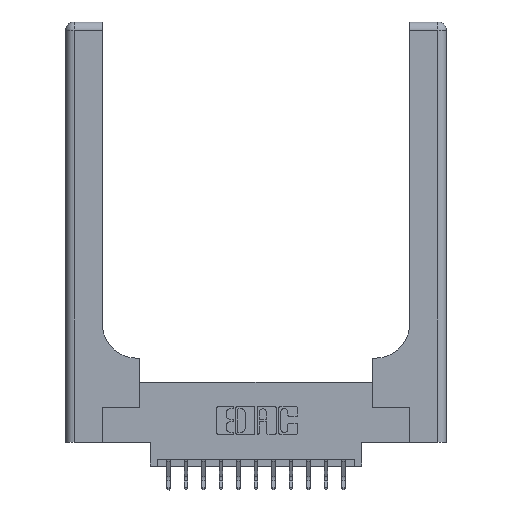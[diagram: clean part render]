
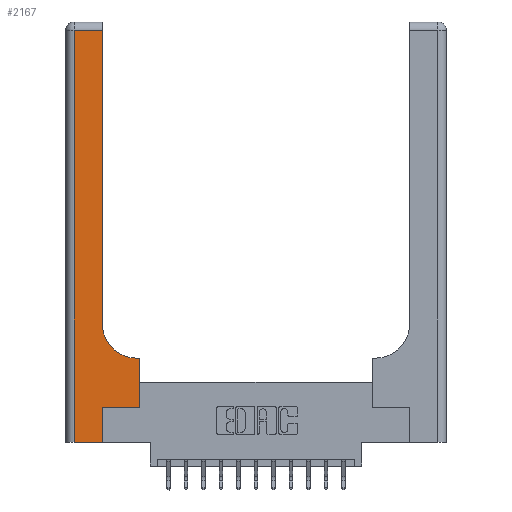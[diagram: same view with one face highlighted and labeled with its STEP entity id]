
A CAD part, top view. The second image highlights one B-rep face of the part: STEP entity #2167.
In plain terms, the highlighted planar face has unit normal (0, 0, 1).
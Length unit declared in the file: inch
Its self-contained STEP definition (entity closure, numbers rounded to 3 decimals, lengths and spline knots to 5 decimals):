
#130 = LINE ( 'NONE', #3756, #10154 ) ;
#184 = CARTESIAN_POINT ( 'NONE',  ( 0.265, 0., 0.37 ) ) ;
#485 = CARTESIAN_POINT ( 'NONE',  ( 0.06, 3., 0.37 ) ) ;
#632 = CARTESIAN_POINT ( 'NONE',  ( 0.06, 2.94, 0.37 ) ) ;
#794 = DIRECTION ( 'NONE',  ( 0., 0., -1. ) ) ;
#854 = EDGE_LOOP ( 'NONE', ( #14864, #3036, #4388, #7846, #2228, #5506, #1753, #13239, #13585 ) ) ;
#1024 = EDGE_CURVE ( 'NONE', #13866, #11968, #15956, .T. ) ;
#1251 = CARTESIAN_POINT ( 'NONE',  ( 0.51, 0.6, 0.37 ) ) ;
#1738 = VERTEX_POINT ( 'NONE', #6323 ) ;
#1753 = ORIENTED_EDGE ( 'NONE', *, *, #13059, .T. ) ;
#2167 = ADVANCED_FACE ( 'NONE', ( #7966 ), #7326, .F. ) ;
#2228 = ORIENTED_EDGE ( 'NONE', *, *, #11933, .T. ) ;
#2257 = VERTEX_POINT ( 'NONE', #12756 ) ;
#2336 = VERTEX_POINT ( 'NONE', #15504 ) ;
#2717 = LINE ( 'NONE', #6917, #5769 ) ;
#2719 = VECTOR ( 'NONE', #6341, 39.37008 ) ;
#2780 = DIRECTION ( 'NONE',  ( 1., 0., 0. ) ) ;
#2996 = DIRECTION ( 'NONE',  ( -1., 0., 0. ) ) ;
#3036 = ORIENTED_EDGE ( 'NONE', *, *, #8027, .T. ) ;
#3420 = LINE ( 'NONE', #8234, #6069 ) ;
#3756 = CARTESIAN_POINT ( 'NONE',  ( 0.26, 3., 0.37 ) ) ;
#4343 = VERTEX_POINT ( 'NONE', #8434 ) ;
#4388 = ORIENTED_EDGE ( 'NONE', *, *, #1024, .T. ) ;
#4531 = DIRECTION ( 'NONE',  ( 0., 0., -1. ) ) ;
#5058 = CARTESIAN_POINT ( 'NONE',  ( 0.528, 0.25, 0.37 ) ) ;
#5084 = DIRECTION ( 'NONE',  ( 0., 1., 0. ) ) ;
#5220 = VECTOR ( 'NONE', #5369, 39.37008 ) ;
#5369 = DIRECTION ( 'NONE',  ( 0., 1., 0. ) ) ;
#5506 = ORIENTED_EDGE ( 'NONE', *, *, #14210, .T. ) ;
#5613 = LINE ( 'NONE', #184, #5220 ) ;
#5717 = DIRECTION ( 'NONE',  ( 0., -1., 0. ) ) ;
#5769 = VECTOR ( 'NONE', #2996, 39.37008 ) ;
#5957 = LINE ( 'NONE', #11010, #15924 ) ;
#6069 = VECTOR ( 'NONE', #6934, 39.37008 ) ;
#6307 = EDGE_CURVE ( 'NONE', #7833, #2257, #9080, .T. ) ;
#6323 = CARTESIAN_POINT ( 'NONE',  ( 0.265, 0.25, 0.37 ) ) ;
#6341 = DIRECTION ( 'NONE',  ( 0., 1., 0. ) ) ;
#6917 = CARTESIAN_POINT ( 'NONE',  ( 0., 2.94, 0.37 ) ) ;
#6934 = DIRECTION ( 'NONE',  ( 1., 0., 0. ) ) ;
#7326 = PLANE ( 'NONE',  #12586 ) ;
#7833 = VERTEX_POINT ( 'NONE', #1251 ) ;
#7846 = ORIENTED_EDGE ( 'NONE', *, *, #10429, .T. ) ;
#7966 = FACE_OUTER_BOUND ( 'NONE', #854, .T. ) ;
#8027 = EDGE_CURVE ( 'NONE', #9971, #13866, #2717, .T. ) ;
#8234 = CARTESIAN_POINT ( 'NONE',  ( 0., 0., 0.37 ) ) ;
#8434 = CARTESIAN_POINT ( 'NONE',  ( 0.265, 0., 0.37 ) ) ;
#9080 = CIRCLE ( 'NONE', #16508, 0.25 ) ;
#9444 = VECTOR ( 'NONE', #5717, 39.37008 ) ;
#9609 = VECTOR ( 'NONE', #2780, 39.37008 ) ;
#9734 = DIRECTION ( 'NONE',  ( -1., 0., 0. ) ) ;
#9934 = DIRECTION ( 'NONE',  ( -1., 0., 0. ) ) ;
#9971 = VERTEX_POINT ( 'NONE', #16212 ) ;
#10154 = VECTOR ( 'NONE', #5084, 39.37008 ) ;
#10429 = EDGE_CURVE ( 'NONE', #11968, #4343, #3420, .T. ) ;
#11010 = CARTESIAN_POINT ( 'NONE',  ( 0.26, 0.6, 0.37 ) ) ;
#11933 = EDGE_CURVE ( 'NONE', #4343, #1738, #5613, .T. ) ;
#11968 = VERTEX_POINT ( 'NONE', #13333 ) ;
#12345 = CARTESIAN_POINT ( 'NONE',  ( 0.51, 0.85, 0.37 ) ) ;
#12586 = AXIS2_PLACEMENT_3D ( 'NONE', #16417, #794, #9934 ) ;
#12710 = LINE ( 'NONE', #14447, #9609 ) ;
#12756 = CARTESIAN_POINT ( 'NONE',  ( 0.26, 0.85, 0.37 ) ) ;
#13059 = EDGE_CURVE ( 'NONE', #14156, #2336, #13129, .T. ) ;
#13129 = LINE ( 'NONE', #5058, #2719 ) ;
#13239 = ORIENTED_EDGE ( 'NONE', *, *, #14462, .T. ) ;
#13333 = CARTESIAN_POINT ( 'NONE',  ( 0.06, 0., 0.37 ) ) ;
#13585 = ORIENTED_EDGE ( 'NONE', *, *, #6307, .T. ) ;
#13633 = DIRECTION ( 'NONE',  ( 1., 0., 0. ) ) ;
#13866 = VERTEX_POINT ( 'NONE', #632 ) ;
#14156 = VERTEX_POINT ( 'NONE', #16778 ) ;
#14210 = EDGE_CURVE ( 'NONE', #1738, #14156, #12710, .T. ) ;
#14447 = CARTESIAN_POINT ( 'NONE',  ( 0.265, 0.25, 0.37 ) ) ;
#14462 = EDGE_CURVE ( 'NONE', #2336, #7833, #5957, .T. ) ;
#14864 = ORIENTED_EDGE ( 'NONE', *, *, #16874, .T. ) ;
#15504 = CARTESIAN_POINT ( 'NONE',  ( 0.528, 0.6, 0.37 ) ) ;
#15924 = VECTOR ( 'NONE', #9734, 39.37008 ) ;
#15956 = LINE ( 'NONE', #485, #9444 ) ;
#16212 = CARTESIAN_POINT ( 'NONE',  ( 0.26, 2.94, 0.37 ) ) ;
#16417 = CARTESIAN_POINT ( 'NONE',  ( 0., 3., 0.37 ) ) ;
#16508 = AXIS2_PLACEMENT_3D ( 'NONE', #12345, #4531, #13633 ) ;
#16778 = CARTESIAN_POINT ( 'NONE',  ( 0.528, 0.25, 0.37 ) ) ;
#16874 = EDGE_CURVE ( 'NONE', #2257, #9971, #130, .T. ) ;
